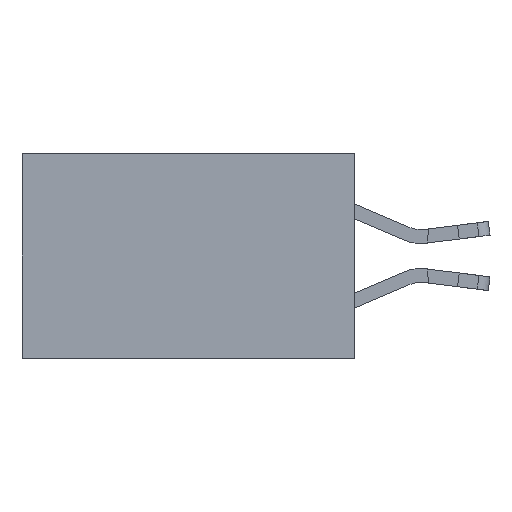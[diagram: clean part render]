
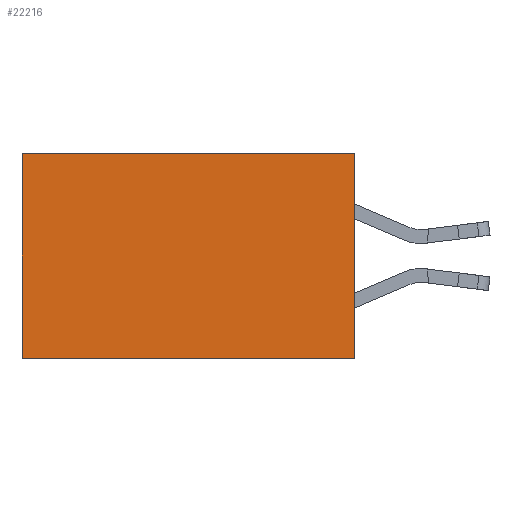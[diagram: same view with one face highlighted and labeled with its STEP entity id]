
A CAD part, left-side view. The second image highlights one B-rep face of the part: STEP entity #22216.
In plain terms, the highlighted planar face has unit normal (-1, 0, 0).
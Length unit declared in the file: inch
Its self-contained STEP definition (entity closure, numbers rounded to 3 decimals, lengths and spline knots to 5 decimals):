
#226 = CARTESIAN_POINT ( 'NONE',  ( 0.298, 0., -0.37 ) ) ;
#1180 = DIRECTION ( 'NONE',  ( 1., 0., 0. ) ) ;
#2462 = CARTESIAN_POINT ( 'NONE',  ( 0.298, 0., 0. ) ) ;
#2795 = EDGE_CURVE ( 'NONE', #7747, #4251, #13998, .T. ) ;
#2819 = AXIS2_PLACEMENT_3D ( 'NONE', #24780, #1180, #14984 ) ;
#3052 = ORIENTED_EDGE ( 'NONE', *, *, #15361, .T. ) ;
#3626 = CARTESIAN_POINT ( 'NONE',  ( 0.298, 0., -0.37 ) ) ;
#4251 = VERTEX_POINT ( 'NONE', #23477 ) ;
#4268 = CARTESIAN_POINT ( 'NONE',  ( 0.298, 0., 0. ) ) ;
#5684 = FACE_OUTER_BOUND ( 'NONE', #15749, .T. ) ;
#6250 = DIRECTION ( 'NONE',  ( 0., 0., -1. ) ) ;
#7747 = VERTEX_POINT ( 'NONE', #2462 ) ;
#8791 = VECTOR ( 'NONE', #15464, 39.37008 ) ;
#9501 = VERTEX_POINT ( 'NONE', #226 ) ;
#9568 = VERTEX_POINT ( 'NONE', #18179 ) ;
#10350 = CARTESIAN_POINT ( 'NONE',  ( 0.298, 0.6, 0. ) ) ;
#10712 = DIRECTION ( 'NONE',  ( 0., 1., 0. ) ) ;
#11084 = EDGE_CURVE ( 'NONE', #9501, #9568, #14046, .T. ) ;
#11238 = ORIENTED_EDGE ( 'NONE', *, *, #2795, .T. ) ;
#12241 = ORIENTED_EDGE ( 'NONE', *, *, #11084, .F. ) ;
#13401 = VECTOR ( 'NONE', #10712, 39.37008 ) ;
#13945 = LINE ( 'NONE', #10350, #18581 ) ;
#13998 = LINE ( 'NONE', #18396, #13401 ) ;
#14046 = LINE ( 'NONE', #3626, #8791 ) ;
#14331 = DIRECTION ( 'NONE',  ( 0., 0., -1. ) ) ;
#14984 = DIRECTION ( 'NONE',  ( 0., 0., -1. ) ) ;
#15361 = EDGE_CURVE ( 'NONE', #4251, #9568, #13945, .T. ) ;
#15464 = DIRECTION ( 'NONE',  ( 0., 1., 0. ) ) ;
#15749 = EDGE_LOOP ( 'NONE', ( #3052, #12241, #16879, #11238 ) ) ;
#16879 = ORIENTED_EDGE ( 'NONE', *, *, #17651, .F. ) ;
#17651 = EDGE_CURVE ( 'NONE', #7747, #9501, #22465, .T. ) ;
#18179 = CARTESIAN_POINT ( 'NONE',  ( 0.298, 0.6, -0.37 ) ) ;
#18396 = CARTESIAN_POINT ( 'NONE',  ( 0.298, 0., 0. ) ) ;
#18581 = VECTOR ( 'NONE', #14331, 39.37008 ) ;
#21847 = VECTOR ( 'NONE', #6250, 39.37008 ) ;
#22216 = ADVANCED_FACE ( 'NONE', ( #5684 ), #24703, .F. ) ;
#22465 = LINE ( 'NONE', #4268, #21847 ) ;
#23477 = CARTESIAN_POINT ( 'NONE',  ( 0.298, 0.6, 0. ) ) ;
#24703 = PLANE ( 'NONE',  #2819 ) ;
#24780 = CARTESIAN_POINT ( 'NONE',  ( 0.298, 0., 0. ) ) ;
